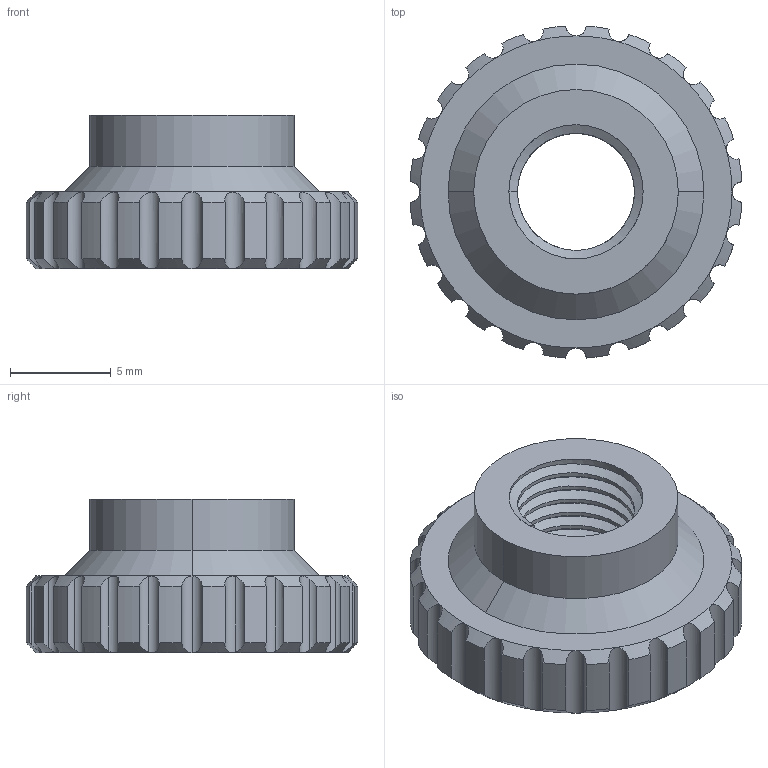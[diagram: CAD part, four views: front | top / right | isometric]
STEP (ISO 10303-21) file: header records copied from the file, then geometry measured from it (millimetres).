
FILE_DESCRIPTION (( 'STEP AP203' ), '1' );
FILE_NAME ('AF-WF-MI-PRT-004-STEP.STEP', '2020-07-21T23:39:29', ( '' ), ( '' ), 'SwSTEP 2.0', 'SolidWorks 2018', '' );
FILE_SCHEMA (( 'CONFIG_CONTROL_DESIGN' ));
Length unit declared in the file: inch
Products named in the file (1): AF-WF-MI-PRT-004-STEP
Bounding box: 16.48 x 16.48 x 7.62 mm (x, y, z)
Volume: 877.1 mm3; surface area: 900.9 mm2
Topology: 1 solids, 1 shells, 138 faces, 350 edges, 215 vertices
Faces by surface type: cylinder 81, cone 50, plane 4, bspline 3
Entity records: 6188 total; most frequent: CARTESIAN_POINT 3080, ORIENTED_EDGE 700, DIRECTION 568, EDGE_CURVE 350, AXIS2_PLACEMENT_3D 241, VERTEX_POINT 215, EDGE_LOOP 141, ADVANCED_FACE 138
